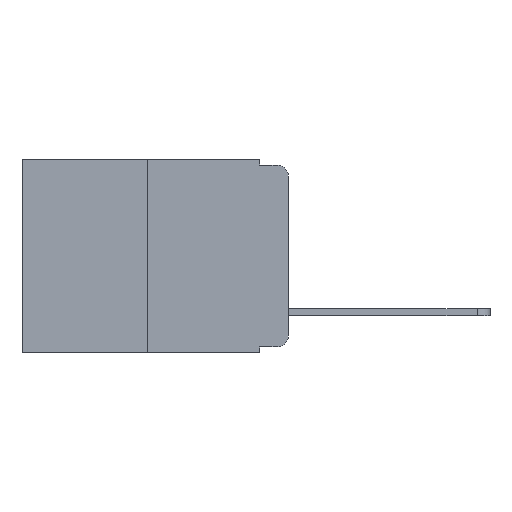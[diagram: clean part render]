
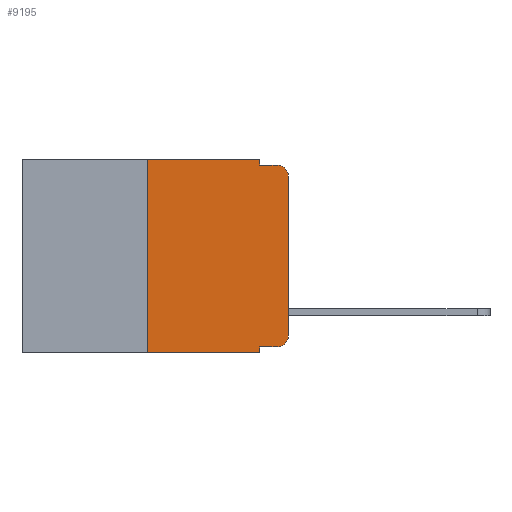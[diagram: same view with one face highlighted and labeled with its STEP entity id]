
A CAD part, left-side view. The second image highlights one B-rep face of the part: STEP entity #9195.
In plain terms, the highlighted planar face has unit normal (-1, 0, 0).
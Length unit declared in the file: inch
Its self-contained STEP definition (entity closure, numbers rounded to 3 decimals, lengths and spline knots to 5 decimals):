
#95 = LINE ( 'NONE', #8650, #4224 ) ;
#298 = VERTEX_POINT ( 'NONE', #919 ) ;
#361 = VECTOR ( 'NONE', #10110, 39.37008 ) ;
#466 = EDGE_CURVE ( 'NONE', #7531, #298, #2421, .T. ) ;
#489 = DIRECTION ( 'NONE',  ( -1., 0., 0. ) ) ;
#527 = DIRECTION ( 'NONE',  ( 0., 0., -1. ) ) ;
#547 = DIRECTION ( 'NONE',  ( 0., 0., -1. ) ) ;
#555 = DIRECTION ( 'NONE',  ( 0., 0., -1. ) ) ;
#613 = VERTEX_POINT ( 'NONE', #10272 ) ;
#684 = VERTEX_POINT ( 'NONE', #9343 ) ;
#836 = DIRECTION ( 'NONE',  ( 0., 0., 1. ) ) ;
#919 = CARTESIAN_POINT ( 'NONE',  ( 0., 0.02, -0.01 ) ) ;
#987 = AXIS2_PLACEMENT_3D ( 'NONE', #2294, #5760, #555 ) ;
#1649 = EDGE_CURVE ( 'NONE', #613, #298, #8943, .T. ) ;
#1708 = DIRECTION ( 'NONE',  ( 0., -1., 0. ) ) ;
#1902 = EDGE_CURVE ( 'NONE', #10517, #7531, #7931, .T. ) ;
#1946 = ORIENTED_EDGE ( 'NONE', *, *, #1649, .T. ) ;
#2122 = AXIS2_PLACEMENT_3D ( 'NONE', #3233, #489, #547 ) ;
#2173 = CARTESIAN_POINT ( 'NONE',  ( 0., 0.02, -0.333 ) ) ;
#2269 = AXIS2_PLACEMENT_3D ( 'NONE', #2449, #3756, #9160 ) ;
#2283 = CIRCLE ( 'NONE', #2269, 0.02 ) ;
#2294 = CARTESIAN_POINT ( 'NONE',  ( 0., 0.473, 0. ) ) ;
#2421 = LINE ( 'NONE', #10506, #361 ) ;
#2449 = CARTESIAN_POINT ( 'NONE',  ( 0., 0.02, -0.313 ) ) ;
#2501 = EDGE_CURVE ( 'NONE', #3389, #5476, #2283, .T. ) ;
#2800 = CARTESIAN_POINT ( 'NONE',  ( 0., 0.473, -0.343 ) ) ;
#3069 = VECTOR ( 'NONE', #5393, 39.37008 ) ;
#3098 = CARTESIAN_POINT ( 'NONE',  ( 0., 0.051, 0. ) ) ;
#3233 = CARTESIAN_POINT ( 'NONE',  ( 0., 0.02, -0.03 ) ) ;
#3234 = VECTOR ( 'NONE', #1708, 39.37008 ) ;
#3379 = CARTESIAN_POINT ( 'NONE',  ( 0., 0., 0. ) ) ;
#3389 = VERTEX_POINT ( 'NONE', #2173 ) ;
#3401 = LINE ( 'NONE', #6916, #9725 ) ;
#3490 = CARTESIAN_POINT ( 'NONE',  ( 0., 0., -0.313 ) ) ;
#3542 = ORIENTED_EDGE ( 'NONE', *, *, #4280, .F. ) ;
#3627 = FACE_OUTER_BOUND ( 'NONE', #5000, .T. ) ;
#3756 = DIRECTION ( 'NONE',  ( -1., 0., 0. ) ) ;
#3967 = LINE ( 'NONE', #3379, #5977 ) ;
#3987 = CARTESIAN_POINT ( 'NONE',  ( 0., 0.051, 0. ) ) ;
#4224 = VECTOR ( 'NONE', #9368, 39.37008 ) ;
#4280 = EDGE_CURVE ( 'NONE', #5339, #10517, #3401, .T. ) ;
#4637 = ORIENTED_EDGE ( 'NONE', *, *, #2501, .T. ) ;
#4883 = ORIENTED_EDGE ( 'NONE', *, *, #466, .F. ) ;
#4930 = PLANE ( 'NONE',  #987 ) ;
#5000 = EDGE_LOOP ( 'NONE', ( #8410, #1946, #4883, #7923, #3542, #5675, #5762, #5477, #5340, #4637 ) ) ;
#5339 = VERTEX_POINT ( 'NONE', #7515 ) ;
#5340 = ORIENTED_EDGE ( 'NONE', *, *, #8118, .T. ) ;
#5393 = DIRECTION ( 'NONE',  ( 0., 0., -1. ) ) ;
#5476 = VERTEX_POINT ( 'NONE', #3490 ) ;
#5477 = ORIENTED_EDGE ( 'NONE', *, *, #6447, .F. ) ;
#5675 = ORIENTED_EDGE ( 'NONE', *, *, #7143, .F. ) ;
#5760 = DIRECTION ( 'NONE',  ( 1., 0., 0. ) ) ;
#5762 = ORIENTED_EDGE ( 'NONE', *, *, #9526, .T. ) ;
#5977 = VECTOR ( 'NONE', #836, 39.37008 ) ;
#6425 = LINE ( 'NONE', #2800, #10134 ) ;
#6447 = EDGE_CURVE ( 'NONE', #7636, #9837, #10302, .T. ) ;
#6683 = DIRECTION ( 'NONE',  ( 0., -1., 0. ) ) ;
#6916 = CARTESIAN_POINT ( 'NONE',  ( 0., 0.473, 0. ) ) ;
#6987 = DIRECTION ( 'NONE',  ( 0., -1., 0. ) ) ;
#7143 = EDGE_CURVE ( 'NONE', #684, #5339, #95, .T. ) ;
#7168 = CARTESIAN_POINT ( 'NONE',  ( 0., 0.051, -0.343 ) ) ;
#7441 = EDGE_CURVE ( 'NONE', #5476, #613, #3967, .T. ) ;
#7515 = CARTESIAN_POINT ( 'NONE',  ( 0., 0.25, 0. ) ) ;
#7529 = CARTESIAN_POINT ( 'NONE',  ( 0., 0.051, -0.333 ) ) ;
#7531 = VERTEX_POINT ( 'NONE', #10552 ) ;
#7636 = VERTEX_POINT ( 'NONE', #8421 ) ;
#7899 = CARTESIAN_POINT ( 'NONE',  ( 0., 0.051, 0. ) ) ;
#7923 = ORIENTED_EDGE ( 'NONE', *, *, #1902, .F. ) ;
#7931 = LINE ( 'NONE', #3987, #3069 ) ;
#8118 = EDGE_CURVE ( 'NONE', #7636, #3389, #9584, .T. ) ;
#8336 = VECTOR ( 'NONE', #527, 39.37008 ) ;
#8410 = ORIENTED_EDGE ( 'NONE', *, *, #7441, .T. ) ;
#8421 = CARTESIAN_POINT ( 'NONE',  ( 0., 0.051, -0.333 ) ) ;
#8650 = CARTESIAN_POINT ( 'NONE',  ( 0., 0.25, 0. ) ) ;
#8943 = CIRCLE ( 'NONE', #2122, 0.02 ) ;
#9160 = DIRECTION ( 'NONE',  ( 0., 0., -1. ) ) ;
#9195 = ADVANCED_FACE ( 'NONE', ( #3627 ), #4930, .F. ) ;
#9343 = CARTESIAN_POINT ( 'NONE',  ( 0., 0.25, -0.343 ) ) ;
#9368 = DIRECTION ( 'NONE',  ( 0., 0., 1. ) ) ;
#9526 = EDGE_CURVE ( 'NONE', #684, #9837, #6425, .T. ) ;
#9584 = LINE ( 'NONE', #7529, #3234 ) ;
#9725 = VECTOR ( 'NONE', #6683, 39.37008 ) ;
#9837 = VERTEX_POINT ( 'NONE', #7168 ) ;
#10110 = DIRECTION ( 'NONE',  ( 0., -1., 0. ) ) ;
#10134 = VECTOR ( 'NONE', #6987, 39.37008 ) ;
#10272 = CARTESIAN_POINT ( 'NONE',  ( 0., 0., -0.03 ) ) ;
#10302 = LINE ( 'NONE', #3098, #8336 ) ;
#10506 = CARTESIAN_POINT ( 'NONE',  ( 0., 0.051, -0.01 ) ) ;
#10517 = VERTEX_POINT ( 'NONE', #7899 ) ;
#10552 = CARTESIAN_POINT ( 'NONE',  ( 0., 0.051, -0.01 ) ) ;
